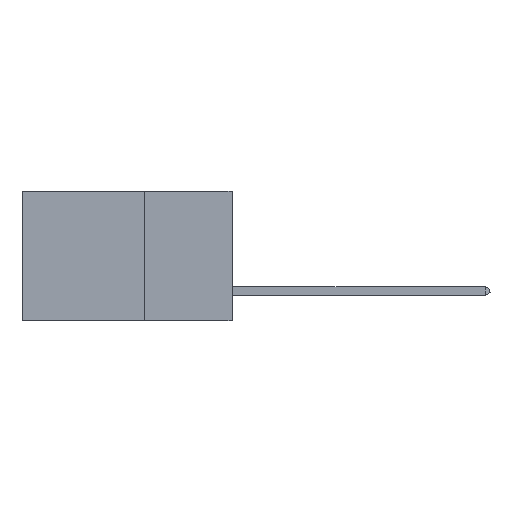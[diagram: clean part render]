
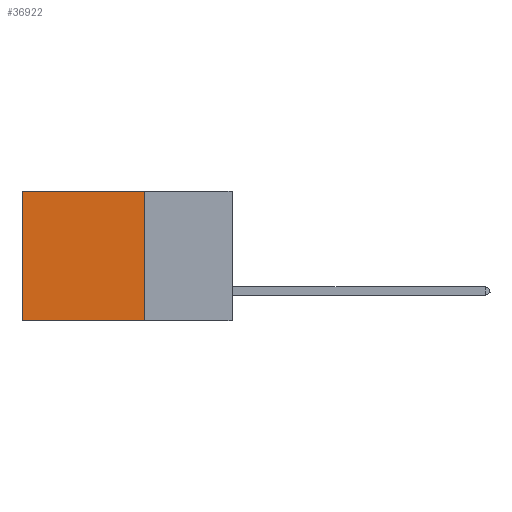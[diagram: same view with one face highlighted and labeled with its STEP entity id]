
A CAD part, left-side view. The second image highlights one B-rep face of the part: STEP entity #36922.
In plain terms, the highlighted planar face has unit normal (-1, 0, 0).
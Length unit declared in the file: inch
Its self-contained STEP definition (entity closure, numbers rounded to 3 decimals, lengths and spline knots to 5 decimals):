
#105 = DIRECTION ( 'NONE',  ( 0., 1., 0. ) ) ;
#1161 = CARTESIAN_POINT ( 'NONE',  ( 0.2875, 0.6, 0. ) ) ;
#2241 = AXIS2_PLACEMENT_3D ( 'NONE', #43154, #7267, #5977 ) ;
#2302 = VECTOR ( 'NONE', #25477, 39.37008 ) ;
#3347 = VERTEX_POINT ( 'NONE', #40898 ) ;
#4390 = CARTESIAN_POINT ( 'NONE',  ( 0.2875, 0.25, 0. ) ) ;
#5977 = DIRECTION ( 'NONE',  ( 0., 0., -1. ) ) ;
#6017 = EDGE_LOOP ( 'NONE', ( #21390, #37650, #23793, #9716 ) ) ;
#6947 = VERTEX_POINT ( 'NONE', #30552 ) ;
#7255 = EDGE_CURVE ( 'NONE', #18673, #3347, #30438, .T. ) ;
#7267 = DIRECTION ( 'NONE',  ( 1., 0., 0. ) ) ;
#7539 = CARTESIAN_POINT ( 'NONE',  ( 0.2875, 0.25, 0. ) ) ;
#8297 = EDGE_CURVE ( 'NONE', #23052, #6947, #42965, .T. ) ;
#8820 = PLANE ( 'NONE',  #2241 ) ;
#9716 = ORIENTED_EDGE ( 'NONE', *, *, #22823, .T. ) ;
#10416 = EDGE_CURVE ( 'NONE', #6947, #3347, #21359, .T. ) ;
#11310 = VECTOR ( 'NONE', #34210, 39.37008 ) ;
#18673 = VERTEX_POINT ( 'NONE', #33305 ) ;
#19016 = LINE ( 'NONE', #4390, #37047 ) ;
#21359 = LINE ( 'NONE', #32456, #44655 ) ;
#21390 = ORIENTED_EDGE ( 'NONE', *, *, #7255, .T. ) ;
#22823 = EDGE_CURVE ( 'NONE', #23052, #18673, #19016, .T. ) ;
#23052 = VERTEX_POINT ( 'NONE', #45213 ) ;
#23793 = ORIENTED_EDGE ( 'NONE', *, *, #8297, .F. ) ;
#25477 = DIRECTION ( 'NONE',  ( 0., 0., -1. ) ) ;
#28740 = FACE_OUTER_BOUND ( 'NONE', #6017, .T. ) ;
#29190 = DIRECTION ( 'NONE',  ( 0., 1., 0. ) ) ;
#30438 = LINE ( 'NONE', #1161, #11310 ) ;
#30552 = CARTESIAN_POINT ( 'NONE',  ( 0.2875, 0.25, -0.37 ) ) ;
#32456 = CARTESIAN_POINT ( 'NONE',  ( 0.2875, 0.25, -0.37 ) ) ;
#33305 = CARTESIAN_POINT ( 'NONE',  ( 0.2875, 0.6, 0. ) ) ;
#34210 = DIRECTION ( 'NONE',  ( 0., 0., -1. ) ) ;
#36922 = ADVANCED_FACE ( 'NONE', ( #28740 ), #8820, .F. ) ;
#37047 = VECTOR ( 'NONE', #29190, 39.37008 ) ;
#37650 = ORIENTED_EDGE ( 'NONE', *, *, #10416, .F. ) ;
#40898 = CARTESIAN_POINT ( 'NONE',  ( 0.2875, 0.6, -0.37 ) ) ;
#42965 = LINE ( 'NONE', #7539, #2302 ) ;
#43154 = CARTESIAN_POINT ( 'NONE',  ( 0.2875, 0.25, 0. ) ) ;
#44655 = VECTOR ( 'NONE', #105, 39.37008 ) ;
#45213 = CARTESIAN_POINT ( 'NONE',  ( 0.2875, 0.25, 0. ) ) ;
